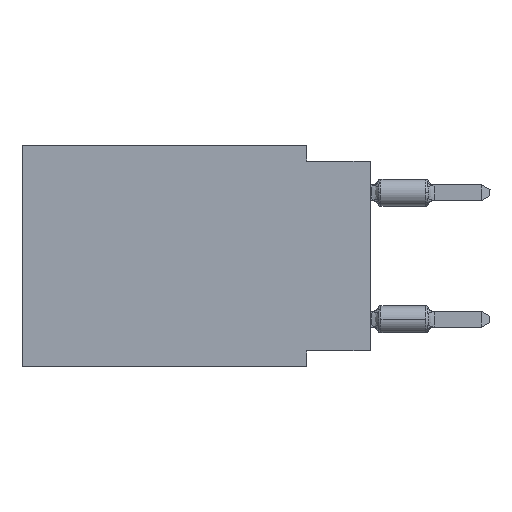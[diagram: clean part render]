
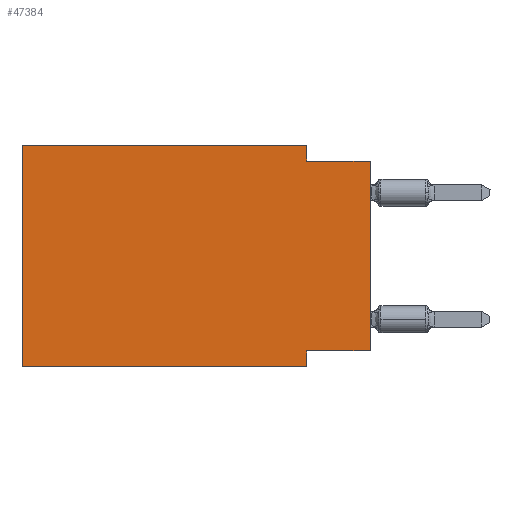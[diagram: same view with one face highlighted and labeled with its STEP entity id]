
A CAD part, left-side view. The second image highlights one B-rep face of the part: STEP entity #47384.
In plain terms, the highlighted planar face has unit normal (-1, 0, 0).
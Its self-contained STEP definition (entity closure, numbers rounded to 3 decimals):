
#1913 = CARTESIAN_POINT ( 'NONE',  ( 0., 13.97, -8.89 ) ) ;
#2303 = EDGE_CURVE ( 'NONE', #48451, #45207, #34323, .T. ) ;
#3539 = ORIENTED_EDGE ( 'NONE', *, *, #23397, .F. ) ;
#3996 = VERTEX_POINT ( 'NONE', #24948 ) ;
#4085 = FACE_OUTER_BOUND ( 'NONE', #28194, .T. ) ;
#4858 = DIRECTION ( 'NONE',  ( 0., 0., 1. ) ) ;
#5757 = AXIS2_PLACEMENT_3D ( 'NONE', #39903, #16527, #11711 ) ;
#9101 = ORIENTED_EDGE ( 'NONE', *, *, #27960, .F. ) ;
#9326 = EDGE_CURVE ( 'NONE', #22862, #42034, #13172, .T. ) ;
#10744 = CARTESIAN_POINT ( 'NONE',  ( 0., 2.54, -8.255 ) ) ;
#11177 = DIRECTION ( 'NONE',  ( 0., -1., 0. ) ) ;
#11349 = DIRECTION ( 'NONE',  ( 0., 0., -1. ) ) ;
#11711 = DIRECTION ( 'NONE',  ( 0., 0., -1. ) ) ;
#12345 = LINE ( 'NONE', #15407, #39614 ) ;
#13172 = LINE ( 'NONE', #21291, #48960 ) ;
#13748 = EDGE_CURVE ( 'NONE', #22862, #45207, #18871, .T. ) ;
#14358 = CARTESIAN_POINT ( 'NONE',  ( 0., 13.97, 0. ) ) ;
#15407 = CARTESIAN_POINT ( 'NONE',  ( 0., 2.54, 0. ) ) ;
#16527 = DIRECTION ( 'NONE',  ( 1., 0., 0. ) ) ;
#18420 = ORIENTED_EDGE ( 'NONE', *, *, #9326, .F. ) ;
#18823 = EDGE_CURVE ( 'NONE', #29917, #33380, #26294, .T. ) ;
#18871 = LINE ( 'NONE', #50147, #28201 ) ;
#19038 = CARTESIAN_POINT ( 'NONE',  ( 0., 13.97, -8.89 ) ) ;
#21291 = CARTESIAN_POINT ( 'NONE',  ( 0., 0., -8.255 ) ) ;
#22474 = EDGE_CURVE ( 'NONE', #33380, #48451, #12345, .T. ) ;
#22799 = VECTOR ( 'NONE', #4858, 1000. ) ;
#22862 = VERTEX_POINT ( 'NONE', #34663 ) ;
#23000 = ORIENTED_EDGE ( 'NONE', *, *, #18823, .F. ) ;
#23397 = EDGE_CURVE ( 'NONE', #42505, #29917, #28988, .T. ) ;
#24948 = CARTESIAN_POINT ( 'NONE',  ( 0., 2.54, -8.89 ) ) ;
#26294 = LINE ( 'NONE', #14358, #40244 ) ;
#26963 = EDGE_CURVE ( 'NONE', #42505, #3996, #44105, .T. ) ;
#27960 = EDGE_CURVE ( 'NONE', #42034, #3996, #30415, .T. ) ;
#28194 = EDGE_LOOP ( 'NONE', ( #32495, #39320, #33077, #23000, #3539, #49610, #9101, #18420 ) ) ;
#28201 = VECTOR ( 'NONE', #34390, 1000. ) ;
#28988 = LINE ( 'NONE', #48311, #22799 ) ;
#29917 = VERTEX_POINT ( 'NONE', #39392 ) ;
#30102 = DIRECTION ( 'NONE',  ( 0., -1., 0. ) ) ;
#30415 = LINE ( 'NONE', #45941, #39750 ) ;
#32495 = ORIENTED_EDGE ( 'NONE', *, *, #13748, .T. ) ;
#33077 = ORIENTED_EDGE ( 'NONE', *, *, #22474, .F. ) ;
#33248 = DIRECTION ( 'NONE',  ( 0., 1., 0. ) ) ;
#33380 = VERTEX_POINT ( 'NONE', #49202 ) ;
#33705 = VECTOR ( 'NONE', #11177, 1000. ) ;
#34323 = LINE ( 'NONE', #46017, #33705 ) ;
#34390 = DIRECTION ( 'NONE',  ( 0., 0., 1. ) ) ;
#34663 = CARTESIAN_POINT ( 'NONE',  ( 0., 0., -8.255 ) ) ;
#34778 = VECTOR ( 'NONE', #36972, 1000. ) ;
#36972 = DIRECTION ( 'NONE',  ( 0., -1., 0. ) ) ;
#38568 = CARTESIAN_POINT ( 'NONE',  ( 0., 2.54, -0.635 ) ) ;
#39320 = ORIENTED_EDGE ( 'NONE', *, *, #2303, .F. ) ;
#39392 = CARTESIAN_POINT ( 'NONE',  ( 0., 13.97, 0. ) ) ;
#39614 = VECTOR ( 'NONE', #47176, 1000. ) ;
#39750 = VECTOR ( 'NONE', #11349, 1000. ) ;
#39903 = CARTESIAN_POINT ( 'NONE',  ( 0., 13.97, 0. ) ) ;
#40244 = VECTOR ( 'NONE', #30102, 1000. ) ;
#42034 = VERTEX_POINT ( 'NONE', #10744 ) ;
#42505 = VERTEX_POINT ( 'NONE', #19038 ) ;
#44105 = LINE ( 'NONE', #1913, #34778 ) ;
#45207 = VERTEX_POINT ( 'NONE', #48212 ) ;
#45941 = CARTESIAN_POINT ( 'NONE',  ( 0., 2.54, -8.89 ) ) ;
#46017 = CARTESIAN_POINT ( 'NONE',  ( 0., 0., -0.635 ) ) ;
#46546 = PLANE ( 'NONE',  #5757 ) ;
#47176 = DIRECTION ( 'NONE',  ( 0., 0., -1. ) ) ;
#47384 = ADVANCED_FACE ( 'NONE', ( #4085 ), #46546, .F. ) ;
#48212 = CARTESIAN_POINT ( 'NONE',  ( 0., 0., -0.635 ) ) ;
#48311 = CARTESIAN_POINT ( 'NONE',  ( 0., 13.97, 0. ) ) ;
#48451 = VERTEX_POINT ( 'NONE', #38568 ) ;
#48960 = VECTOR ( 'NONE', #33248, 1000. ) ;
#49202 = CARTESIAN_POINT ( 'NONE',  ( 0., 2.54, 0. ) ) ;
#49610 = ORIENTED_EDGE ( 'NONE', *, *, #26963, .T. ) ;
#50147 = CARTESIAN_POINT ( 'NONE',  ( 0., 0., 0. ) ) ;
